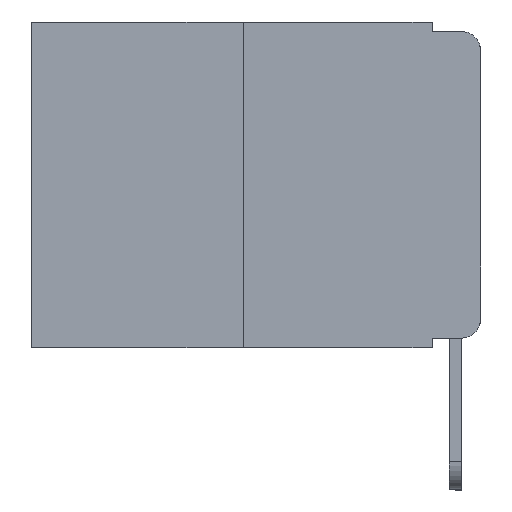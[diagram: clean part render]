
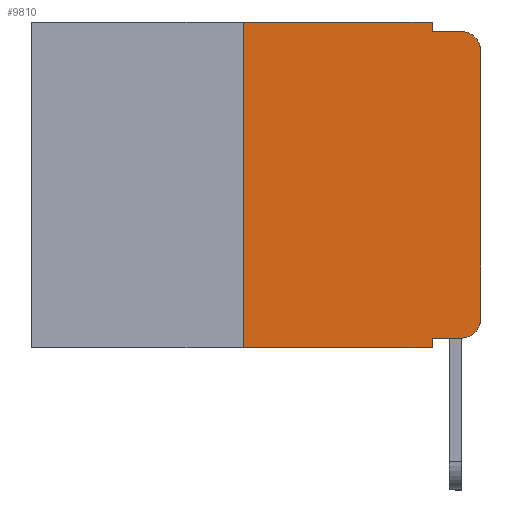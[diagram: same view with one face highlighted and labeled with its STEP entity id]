
A CAD part, left-side view. The second image highlights one B-rep face of the part: STEP entity #9810.
In plain terms, the highlighted planar face has unit normal (-1, 0, 0).
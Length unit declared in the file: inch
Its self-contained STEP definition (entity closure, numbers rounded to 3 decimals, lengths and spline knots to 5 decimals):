
#272 = VERTEX_POINT ( 'NONE', #3895 ) ;
#609 = CARTESIAN_POINT ( 'NONE',  ( 0., 0.051, 0. ) ) ;
#813 = VERTEX_POINT ( 'NONE', #6009 ) ;
#1367 = LINE ( 'NONE', #13491, #6926 ) ;
#1566 = ORIENTED_EDGE ( 'NONE', *, *, #9366, .F. ) ;
#1669 = VERTEX_POINT ( 'NONE', #14224 ) ;
#1756 = CARTESIAN_POINT ( 'NONE',  ( 0., 0.25, 0. ) ) ;
#2245 = DIRECTION ( 'NONE',  ( 0., 0., -1. ) ) ;
#2402 = EDGE_CURVE ( 'NONE', #1669, #12378, #11262, .T. ) ;
#3024 = EDGE_CURVE ( 'NONE', #15332, #813, #4591, .T. ) ;
#3039 = CARTESIAN_POINT ( 'NONE',  ( 0., 0.473, 0. ) ) ;
#3098 = LINE ( 'NONE', #1756, #5477 ) ;
#3378 = CARTESIAN_POINT ( 'NONE',  ( 0., 0.25, 0. ) ) ;
#3540 = CARTESIAN_POINT ( 'NONE',  ( 0., 0.02, -0.03 ) ) ;
#3676 = AXIS2_PLACEMENT_3D ( 'NONE', #3039, #13444, #12429 ) ;
#3895 = CARTESIAN_POINT ( 'NONE',  ( 0., 0.25, -0.343 ) ) ;
#3903 = DIRECTION ( 'NONE',  ( 0., 0., 1. ) ) ;
#3923 = VECTOR ( 'NONE', #5467, 39.37008 ) ;
#4164 = ORIENTED_EDGE ( 'NONE', *, *, #6290, .T. ) ;
#4250 = EDGE_CURVE ( 'NONE', #9073, #15332, #5468, .T. ) ;
#4291 = ORIENTED_EDGE ( 'NONE', *, *, #9078, .T. ) ;
#4591 = LINE ( 'NONE', #8144, #6695 ) ;
#4888 = AXIS2_PLACEMENT_3D ( 'NONE', #3540, #7017, #6801 ) ;
#4927 = VERTEX_POINT ( 'NONE', #12174 ) ;
#5318 = VECTOR ( 'NONE', #3903, 39.37008 ) ;
#5389 = ORIENTED_EDGE ( 'NONE', *, *, #4250, .F. ) ;
#5445 = PLANE ( 'NONE',  #3676 ) ;
#5467 = DIRECTION ( 'NONE',  ( 0., -1., 0. ) ) ;
#5468 = LINE ( 'NONE', #10698, #14263 ) ;
#5477 = VECTOR ( 'NONE', #6509, 39.37008 ) ;
#5782 = ORIENTED_EDGE ( 'NONE', *, *, #7680, .T. ) ;
#6009 = CARTESIAN_POINT ( 'NONE',  ( 0., 0.051, -0.01 ) ) ;
#6290 = EDGE_CURVE ( 'NONE', #272, #12378, #1367, .T. ) ;
#6383 = VERTEX_POINT ( 'NONE', #9127 ) ;
#6509 = DIRECTION ( 'NONE',  ( 0., 0., 1. ) ) ;
#6620 = LINE ( 'NONE', #11341, #3923 ) ;
#6636 = VECTOR ( 'NONE', #12690, 39.37008 ) ;
#6695 = VECTOR ( 'NONE', #2245, 39.37008 ) ;
#6801 = DIRECTION ( 'NONE',  ( 0., 0., -1. ) ) ;
#6926 = VECTOR ( 'NONE', #9829, 39.37008 ) ;
#7015 = CARTESIAN_POINT ( 'NONE',  ( 0., 0.051, -0.333 ) ) ;
#7017 = DIRECTION ( 'NONE',  ( -1., 0., 0. ) ) ;
#7374 = AXIS2_PLACEMENT_3D ( 'NONE', #10160, #14932, #9010 ) ;
#7673 = FACE_OUTER_BOUND ( 'NONE', #10547, .T. ) ;
#7680 = EDGE_CURVE ( 'NONE', #4927, #6383, #9842, .T. ) ;
#7847 = ORIENTED_EDGE ( 'NONE', *, *, #9823, .T. ) ;
#8131 = EDGE_CURVE ( 'NONE', #1669, #14369, #14098, .T. ) ;
#8144 = CARTESIAN_POINT ( 'NONE',  ( 0., 0.051, 0. ) ) ;
#8528 = ORIENTED_EDGE ( 'NONE', *, *, #8131, .T. ) ;
#8840 = ORIENTED_EDGE ( 'NONE', *, *, #2402, .F. ) ;
#9010 = DIRECTION ( 'NONE',  ( 0., 0., -1. ) ) ;
#9073 = VERTEX_POINT ( 'NONE', #3378 ) ;
#9078 = EDGE_CURVE ( 'NONE', #6383, #9887, #14144, .T. ) ;
#9097 = DIRECTION ( 'NONE',  ( 0., 0., -1. ) ) ;
#9127 = CARTESIAN_POINT ( 'NONE',  ( 0., 0., -0.03 ) ) ;
#9366 = EDGE_CURVE ( 'NONE', #813, #9887, #6620, .T. ) ;
#9810 = ADVANCED_FACE ( 'NONE', ( #7673 ), #5445, .F. ) ;
#9823 = EDGE_CURVE ( 'NONE', #14369, #4927, #12095, .T. ) ;
#9829 = DIRECTION ( 'NONE',  ( 0., -1., 0. ) ) ;
#9842 = LINE ( 'NONE', #11312, #5318 ) ;
#9887 = VERTEX_POINT ( 'NONE', #11723 ) ;
#10160 = CARTESIAN_POINT ( 'NONE',  ( 0., 0.02, -0.313 ) ) ;
#10469 = CARTESIAN_POINT ( 'NONE',  ( 0., 0.051, 0. ) ) ;
#10547 = EDGE_LOOP ( 'NONE', ( #5782, #4291, #1566, #15208, #5389, #13619, #4164, #8840, #8528, #7847 ) ) ;
#10698 = CARTESIAN_POINT ( 'NONE',  ( 0., 0.473, 0. ) ) ;
#11262 = LINE ( 'NONE', #609, #14628 ) ;
#11312 = CARTESIAN_POINT ( 'NONE',  ( 0., 0., 0. ) ) ;
#11341 = CARTESIAN_POINT ( 'NONE',  ( 0., 0.051, -0.01 ) ) ;
#11723 = CARTESIAN_POINT ( 'NONE',  ( 0., 0.02, -0.01 ) ) ;
#11998 = CARTESIAN_POINT ( 'NONE',  ( 0., 0.02, -0.333 ) ) ;
#12095 = CIRCLE ( 'NONE', #7374, 0.02 ) ;
#12174 = CARTESIAN_POINT ( 'NONE',  ( 0., 0., -0.313 ) ) ;
#12378 = VERTEX_POINT ( 'NONE', #13810 ) ;
#12429 = DIRECTION ( 'NONE',  ( 0., 0., -1. ) ) ;
#12464 = EDGE_CURVE ( 'NONE', #272, #9073, #3098, .T. ) ;
#12690 = DIRECTION ( 'NONE',  ( 0., -1., 0. ) ) ;
#13444 = DIRECTION ( 'NONE',  ( 1., 0., 0. ) ) ;
#13491 = CARTESIAN_POINT ( 'NONE',  ( 0., 0.473, -0.343 ) ) ;
#13619 = ORIENTED_EDGE ( 'NONE', *, *, #12464, .F. ) ;
#13810 = CARTESIAN_POINT ( 'NONE',  ( 0., 0.051, -0.343 ) ) ;
#14098 = LINE ( 'NONE', #7015, #6636 ) ;
#14144 = CIRCLE ( 'NONE', #4888, 0.02 ) ;
#14224 = CARTESIAN_POINT ( 'NONE',  ( 0., 0.051, -0.333 ) ) ;
#14263 = VECTOR ( 'NONE', #14951, 39.37008 ) ;
#14369 = VERTEX_POINT ( 'NONE', #11998 ) ;
#14628 = VECTOR ( 'NONE', #9097, 39.37008 ) ;
#14932 = DIRECTION ( 'NONE',  ( -1., 0., 0. ) ) ;
#14951 = DIRECTION ( 'NONE',  ( 0., -1., 0. ) ) ;
#15208 = ORIENTED_EDGE ( 'NONE', *, *, #3024, .F. ) ;
#15332 = VERTEX_POINT ( 'NONE', #10469 ) ;
